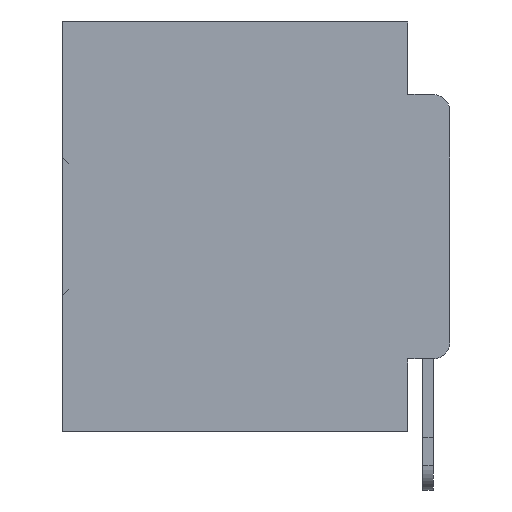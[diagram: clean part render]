
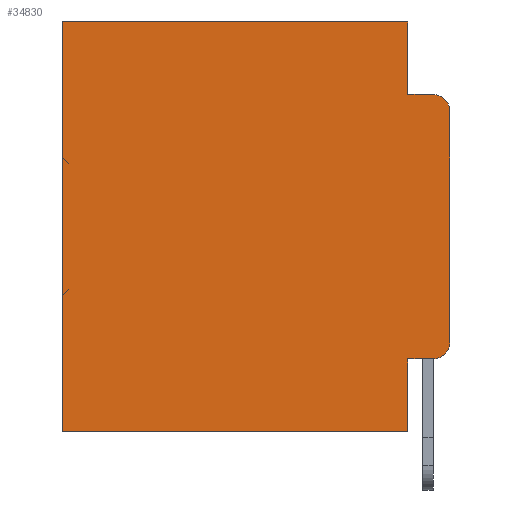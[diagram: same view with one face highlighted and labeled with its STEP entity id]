
A CAD part, left-side view. The second image highlights one B-rep face of the part: STEP entity #34830.
In plain terms, the highlighted planar face has unit normal (-1, 0, 0).
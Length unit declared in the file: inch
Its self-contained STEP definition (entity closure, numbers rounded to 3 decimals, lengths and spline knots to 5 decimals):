
#292 = LINE ( 'NONE', #2360, #22307 ) ;
#402 = ORIENTED_EDGE ( 'NONE', *, *, #21389, .T. ) ;
#870 = ORIENTED_EDGE ( 'NONE', *, *, #32549, .F. ) ;
#952 = ORIENTED_EDGE ( 'NONE', *, *, #5694, .F. ) ;
#1030 = DIRECTION ( 'NONE',  ( 0., 0., -1. ) ) ;
#1104 = VECTOR ( 'NONE', #9628, 39.37008 ) ;
#1476 = ORIENTED_EDGE ( 'NONE', *, *, #31356, .T. ) ;
#1527 = ORIENTED_EDGE ( 'NONE', *, *, #4392, .T. ) ;
#1552 = ORIENTED_EDGE ( 'NONE', *, *, #26379, .T. ) ;
#1674 = EDGE_CURVE ( 'NONE', #26949, #21182, #31456, .T. ) ;
#2360 = CARTESIAN_POINT ( 'NONE',  ( 0.298, 0.051, -0.4115 ) ) ;
#2878 = LINE ( 'NONE', #9761, #31990 ) ;
#3933 = EDGE_CURVE ( 'NONE', #16776, #5674, #32024, .T. ) ;
#4228 = ORIENTED_EDGE ( 'NONE', *, *, #1674, .F. ) ;
#4392 = EDGE_CURVE ( 'NONE', #26949, #32153, #2878, .T. ) ;
#4616 = LINE ( 'NONE', #15518, #26382 ) ;
#5306 = DIRECTION ( 'NONE',  ( 0., -1., 0. ) ) ;
#5398 = CARTESIAN_POINT ( 'NONE',  ( 0.298, 0.051, -0.5 ) ) ;
#5674 = VERTEX_POINT ( 'NONE', #21069 ) ;
#5694 = EDGE_CURVE ( 'NONE', #16115, #18705, #4616, .T. ) ;
#6414 = ORIENTED_EDGE ( 'NONE', *, *, #8521, .T. ) ;
#6735 = CARTESIAN_POINT ( 'NONE',  ( 0.298, 0., -0.5 ) ) ;
#7024 = DIRECTION ( 'NONE',  ( 0., 1., 0. ) ) ;
#8447 = DIRECTION ( 'NONE',  ( 0., 0., -1. ) ) ;
#8521 = EDGE_CURVE ( 'NONE', #16776, #29193, #31688, .T. ) ;
#8789 = ORIENTED_EDGE ( 'NONE', *, *, #19233, .F. ) ;
#8961 = CARTESIAN_POINT ( 'NONE',  ( 0.298, 0.02, -0.4115 ) ) ;
#9628 = DIRECTION ( 'NONE',  ( 0., 1., 0. ) ) ;
#9668 = EDGE_LOOP ( 'NONE', ( #10964, #6414, #8789, #4228, #1527, #402, #870, #952, #1476, #1552 ) ) ;
#9761 = CARTESIAN_POINT ( 'NONE',  ( 0.298, 0., 0. ) ) ;
#9938 = CARTESIAN_POINT ( 'NONE',  ( 0.298, 0.473, -0.5 ) ) ;
#10669 = DIRECTION ( 'NONE',  ( 0., -1., 0. ) ) ;
#10700 = LINE ( 'NONE', #6735, #1104 ) ;
#10964 = ORIENTED_EDGE ( 'NONE', *, *, #3933, .F. ) ;
#11199 = VECTOR ( 'NONE', #10669, 39.37008 ) ;
#11279 = DIRECTION ( 'NONE',  ( 1., 0., 0. ) ) ;
#11705 = CARTESIAN_POINT ( 'NONE',  ( 0.298, 0.473, 0. ) ) ;
#14557 = VERTEX_POINT ( 'NONE', #9938 ) ;
#15518 = CARTESIAN_POINT ( 'NONE',  ( 0.298, 0.051, 0. ) ) ;
#15854 = AXIS2_PLACEMENT_3D ( 'NONE', #16407, #35726, #19262 ) ;
#16115 = VERTEX_POINT ( 'NONE', #27764 ) ;
#16407 = CARTESIAN_POINT ( 'NONE',  ( 0.298, 0.02, -0.3915 ) ) ;
#16776 = VERTEX_POINT ( 'NONE', #19439 ) ;
#17158 = AXIS2_PLACEMENT_3D ( 'NONE', #28102, #11279, #30811 ) ;
#18279 = DIRECTION ( 'NONE',  ( -1., 0., 0. ) ) ;
#18290 = FACE_OUTER_BOUND ( 'NONE', #9668, .T. ) ;
#18350 = DIRECTION ( 'NONE',  ( 0., 0., -1. ) ) ;
#18705 = VERTEX_POINT ( 'NONE', #5398 ) ;
#19233 = EDGE_CURVE ( 'NONE', #21182, #29193, #26178, .T. ) ;
#19262 = DIRECTION ( 'NONE',  ( 0., 0., -1. ) ) ;
#19352 = DIRECTION ( 'NONE',  ( 0., 0., -1. ) ) ;
#19439 = CARTESIAN_POINT ( 'NONE',  ( 0.298, 0., -0.1085 ) ) ;
#20017 = CARTESIAN_POINT ( 'NONE',  ( 0.298, 0.051, 0. ) ) ;
#20310 = LINE ( 'NONE', #11705, #26866 ) ;
#21069 = CARTESIAN_POINT ( 'NONE',  ( 0.298, 0., -0.3915 ) ) ;
#21182 = VERTEX_POINT ( 'NONE', #27826 ) ;
#21389 = EDGE_CURVE ( 'NONE', #32153, #14557, #20310, .T. ) ;
#22054 = CARTESIAN_POINT ( 'NONE',  ( 0.298, 0.051, -0.0885 ) ) ;
#22307 = VECTOR ( 'NONE', #5306, 39.37008 ) ;
#23205 = DIRECTION ( 'NONE',  ( 0., 0., -1. ) ) ;
#24197 = VECTOR ( 'NONE', #8447, 39.37008 ) ;
#24420 = CIRCLE ( 'NONE', #15854, 0.02 ) ;
#24766 = VECTOR ( 'NONE', #19352, 39.37008 ) ;
#26178 = LINE ( 'NONE', #22054, #11199 ) ;
#26379 = EDGE_CURVE ( 'NONE', #34144, #5674, #24420, .T. ) ;
#26382 = VECTOR ( 'NONE', #18350, 39.37008 ) ;
#26866 = VECTOR ( 'NONE', #23205, 39.37008 ) ;
#26949 = VERTEX_POINT ( 'NONE', #20017 ) ;
#27764 = CARTESIAN_POINT ( 'NONE',  ( 0.298, 0.051, -0.4115 ) ) ;
#27826 = CARTESIAN_POINT ( 'NONE',  ( 0.298, 0.051, -0.0885 ) ) ;
#28102 = CARTESIAN_POINT ( 'NONE',  ( 0.298, 0., 0. ) ) ;
#28992 = AXIS2_PLACEMENT_3D ( 'NONE', #34778, #18279, #1030 ) ;
#29193 = VERTEX_POINT ( 'NONE', #33114 ) ;
#29998 = CARTESIAN_POINT ( 'NONE',  ( 0.298, 0.473, 0. ) ) ;
#30101 = PLANE ( 'NONE',  #17158 ) ;
#30811 = DIRECTION ( 'NONE',  ( 0., 0., -1. ) ) ;
#31356 = EDGE_CURVE ( 'NONE', #16115, #34144, #292, .T. ) ;
#31456 = LINE ( 'NONE', #32096, #24197 ) ;
#31688 = CIRCLE ( 'NONE', #28992, 0.02 ) ;
#31990 = VECTOR ( 'NONE', #7024, 39.37008 ) ;
#32024 = LINE ( 'NONE', #35810, #24766 ) ;
#32096 = CARTESIAN_POINT ( 'NONE',  ( 0.298, 0.051, 0. ) ) ;
#32153 = VERTEX_POINT ( 'NONE', #29998 ) ;
#32549 = EDGE_CURVE ( 'NONE', #18705, #14557, #10700, .T. ) ;
#33114 = CARTESIAN_POINT ( 'NONE',  ( 0.298, 0.02, -0.0885 ) ) ;
#34144 = VERTEX_POINT ( 'NONE', #8961 ) ;
#34778 = CARTESIAN_POINT ( 'NONE',  ( 0.298, 0.02, -0.1085 ) ) ;
#34830 = ADVANCED_FACE ( 'NONE', ( #18290 ), #30101, .F. ) ;
#35726 = DIRECTION ( 'NONE',  ( -1., 0., 0. ) ) ;
#35810 = CARTESIAN_POINT ( 'NONE',  ( 0.298, 0., 0. ) ) ;
